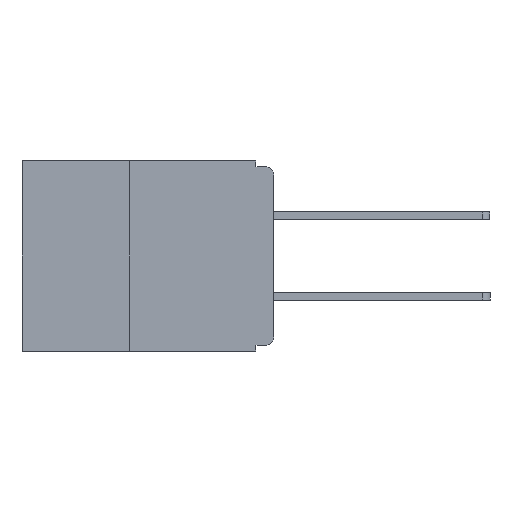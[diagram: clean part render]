
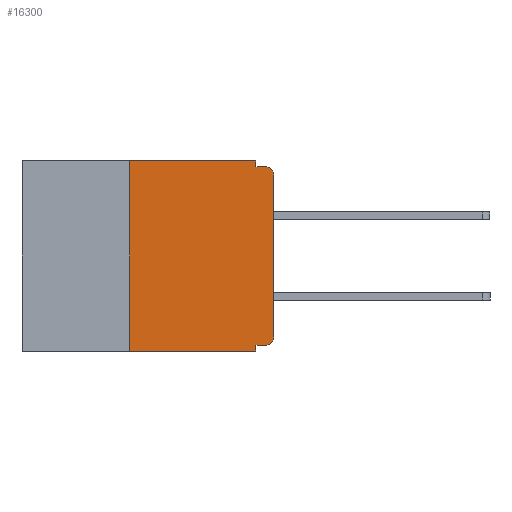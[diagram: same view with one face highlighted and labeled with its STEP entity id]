
A CAD part, left-side view. The second image highlights one B-rep face of the part: STEP entity #16300.
In plain terms, the highlighted planar face has unit normal (-1, 0, 0).
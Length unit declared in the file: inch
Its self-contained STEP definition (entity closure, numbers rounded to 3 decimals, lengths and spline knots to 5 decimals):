
#54 = VERTEX_POINT ( 'NONE', #22718 ) ;
#670 = DIRECTION ( 'NONE',  ( 0., 0., -1. ) ) ;
#898 = CARTESIAN_POINT ( 'NONE',  ( 0., 0.031, -0.33 ) ) ;
#1334 = LINE ( 'NONE', #14141, #17685 ) ;
#1551 = ORIENTED_EDGE ( 'NONE', *, *, #10013, .T. ) ;
#1638 = CARTESIAN_POINT ( 'NONE',  ( 0., 0., 0. ) ) ;
#2374 = LINE ( 'NONE', #15800, #25047 ) ;
#2557 = DIRECTION ( 'NONE',  ( 0., -1., 0. ) ) ;
#2837 = VERTEX_POINT ( 'NONE', #23400 ) ;
#2975 = DIRECTION ( 'NONE',  ( 0., 0., -1. ) ) ;
#2980 = DIRECTION ( 'NONE',  ( -1., 0., 0. ) ) ;
#3000 = CARTESIAN_POINT ( 'NONE',  ( 0., 0.015, -0.305 ) ) ;
#3164 = CARTESIAN_POINT ( 'NONE',  ( 0., 0.031, 0. ) ) ;
#3297 = ORIENTED_EDGE ( 'NONE', *, *, #20544, .F. ) ;
#3452 = CARTESIAN_POINT ( 'NONE',  ( 0., 0.031, -0.33 ) ) ;
#3892 = DIRECTION ( 'NONE',  ( 0., 0., 1. ) ) ;
#3969 = CARTESIAN_POINT ( 'NONE',  ( 0., 0.015, -0.025 ) ) ;
#4128 = EDGE_CURVE ( 'NONE', #14926, #7181, #26477, .T. ) ;
#4586 = EDGE_CURVE ( 'NONE', #18898, #9333, #27070, .T. ) ;
#5216 = CARTESIAN_POINT ( 'NONE',  ( 0., 0.031, -0.32 ) ) ;
#5881 = VERTEX_POINT ( 'NONE', #3452 ) ;
#6217 = DIRECTION ( 'NONE',  ( 0., 0., -1. ) ) ;
#6274 = VERTEX_POINT ( 'NONE', #5216 ) ;
#6802 = VERTEX_POINT ( 'NONE', #7015 ) ;
#6948 = LINE ( 'NONE', #898, #10714 ) ;
#7015 = CARTESIAN_POINT ( 'NONE',  ( 0., 0.25, -0.33 ) ) ;
#7181 = VERTEX_POINT ( 'NONE', #25901 ) ;
#7439 = ORIENTED_EDGE ( 'NONE', *, *, #12986, .F. ) ;
#8160 = VERTEX_POINT ( 'NONE', #23767 ) ;
#8801 = CARTESIAN_POINT ( 'NONE',  ( 0., 0., -0.32 ) ) ;
#9306 = ORIENTED_EDGE ( 'NONE', *, *, #4128, .T. ) ;
#9333 = VERTEX_POINT ( 'NONE', #25845 ) ;
#9513 = CARTESIAN_POINT ( 'NONE',  ( 0., 0.437, 0. ) ) ;
#9782 = DIRECTION ( 'NONE',  ( 0., 0., 1. ) ) ;
#10013 = EDGE_CURVE ( 'NONE', #2837, #54, #22098, .T. ) ;
#10296 = LINE ( 'NONE', #1638, #21338 ) ;
#10714 = VECTOR ( 'NONE', #12058, 39.37008 ) ;
#11130 = EDGE_LOOP ( 'NONE', ( #27780, #1551, #12846, #18595, #21890, #3297, #18384, #12204, #7439, #9306 ) ) ;
#11231 = AXIS2_PLACEMENT_3D ( 'NONE', #3969, #19442, #6217 ) ;
#11241 = VECTOR ( 'NONE', #26267, 39.37008 ) ;
#12049 = DIRECTION ( 'NONE',  ( 0., 0., -1. ) ) ;
#12058 = DIRECTION ( 'NONE',  ( 0., 0., -1. ) ) ;
#12204 = ORIENTED_EDGE ( 'NONE', *, *, #17666, .F. ) ;
#12291 = CARTESIAN_POINT ( 'NONE',  ( 0., 0.437, 0. ) ) ;
#12846 = ORIENTED_EDGE ( 'NONE', *, *, #20392, .F. ) ;
#12986 = EDGE_CURVE ( 'NONE', #14926, #6274, #22262, .T. ) ;
#13463 = CARTESIAN_POINT ( 'NONE',  ( 0., 0.015, -0.32 ) ) ;
#13992 = DIRECTION ( 'NONE',  ( 1., 0., 0. ) ) ;
#14141 = CARTESIAN_POINT ( 'NONE',  ( 0., 0.25, -0.33 ) ) ;
#14926 = VERTEX_POINT ( 'NONE', #13463 ) ;
#15654 = VECTOR ( 'NONE', #27429, 39.37008 ) ;
#15800 = CARTESIAN_POINT ( 'NONE',  ( 0., 0.437, -0.33 ) ) ;
#16300 = ADVANCED_FACE ( 'NONE', ( #28046 ), #26932, .F. ) ;
#16342 = AXIS2_PLACEMENT_3D ( 'NONE', #3000, #2980, #2975 ) ;
#16620 = LINE ( 'NONE', #26569, #27318 ) ;
#16867 = VECTOR ( 'NONE', #12049, 39.37008 ) ;
#17666 = EDGE_CURVE ( 'NONE', #6274, #5881, #6948, .T. ) ;
#17685 = VECTOR ( 'NONE', #9782, 39.37008 ) ;
#18159 = DIRECTION ( 'NONE',  ( 0., -1., 0. ) ) ;
#18384 = ORIENTED_EDGE ( 'NONE', *, *, #19128, .T. ) ;
#18595 = ORIENTED_EDGE ( 'NONE', *, *, #22015, .F. ) ;
#18898 = VERTEX_POINT ( 'NONE', #27071 ) ;
#19128 = EDGE_CURVE ( 'NONE', #6802, #5881, #2374, .T. ) ;
#19442 = DIRECTION ( 'NONE',  ( -1., 0., 0. ) ) ;
#20392 = EDGE_CURVE ( 'NONE', #8160, #54, #16620, .T. ) ;
#20544 = EDGE_CURVE ( 'NONE', #6802, #18898, #1334, .T. ) ;
#21338 = VECTOR ( 'NONE', #3892, 39.37008 ) ;
#21890 = ORIENTED_EDGE ( 'NONE', *, *, #4586, .F. ) ;
#22015 = EDGE_CURVE ( 'NONE', #9333, #8160, #28189, .T. ) ;
#22098 = CIRCLE ( 'NONE', #11231, 0.015 ) ;
#22262 = LINE ( 'NONE', #8801, #11241 ) ;
#22718 = CARTESIAN_POINT ( 'NONE',  ( 0., 0.015, -0.01 ) ) ;
#23400 = CARTESIAN_POINT ( 'NONE',  ( 0., 0., -0.025 ) ) ;
#23767 = CARTESIAN_POINT ( 'NONE',  ( 0., 0.031, -0.01 ) ) ;
#25047 = VECTOR ( 'NONE', #18159, 39.37008 ) ;
#25104 = AXIS2_PLACEMENT_3D ( 'NONE', #9513, #13992, #670 ) ;
#25845 = CARTESIAN_POINT ( 'NONE',  ( 0., 0.031, 0. ) ) ;
#25901 = CARTESIAN_POINT ( 'NONE',  ( 0., 0., -0.305 ) ) ;
#26122 = EDGE_CURVE ( 'NONE', #7181, #2837, #10296, .T. ) ;
#26267 = DIRECTION ( 'NONE',  ( 0., 1., 0. ) ) ;
#26477 = CIRCLE ( 'NONE', #16342, 0.015 ) ;
#26569 = CARTESIAN_POINT ( 'NONE',  ( 0., 0., -0.01 ) ) ;
#26932 = PLANE ( 'NONE',  #25104 ) ;
#27070 = LINE ( 'NONE', #12291, #15654 ) ;
#27071 = CARTESIAN_POINT ( 'NONE',  ( 0., 0.25, 0. ) ) ;
#27318 = VECTOR ( 'NONE', #2557, 39.37008 ) ;
#27429 = DIRECTION ( 'NONE',  ( 0., -1., 0. ) ) ;
#27780 = ORIENTED_EDGE ( 'NONE', *, *, #26122, .T. ) ;
#28046 = FACE_OUTER_BOUND ( 'NONE', #11130, .T. ) ;
#28189 = LINE ( 'NONE', #3164, #16867 ) ;
